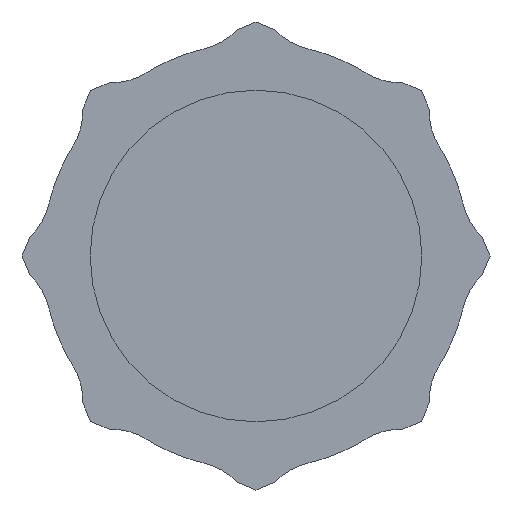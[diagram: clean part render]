
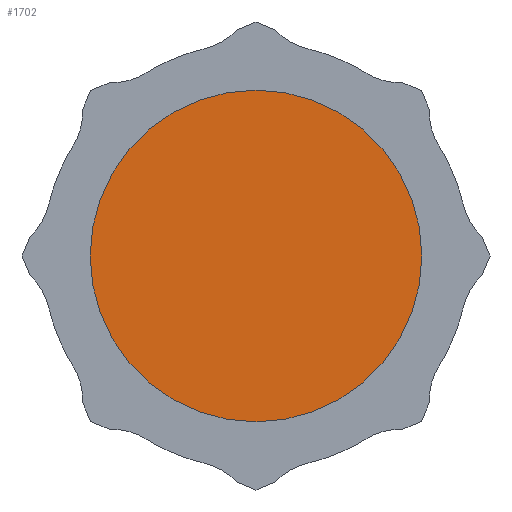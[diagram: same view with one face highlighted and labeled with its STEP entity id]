
A CAD part, front view. The second image highlights one B-rep face of the part: STEP entity #1702.
In plain terms, the highlighted planar face has unit normal (0, -1, 0).
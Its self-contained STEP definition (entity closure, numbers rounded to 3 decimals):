
#25=PLANE('',#1928);
#132=CIRCLE('',#1927,3.125);
#255=FACE_OUTER_BOUND('',#355,.T.);
#355=EDGE_LOOP('',(#1417));
#771=VERTEX_POINT('',#3386);
#1006=EDGE_CURVE('',#771,#771,#132,.T.);
#1417=ORIENTED_EDGE('',*,*,#1006,.T.);
#1702=ADVANCED_FACE('',(#255),#25,.F.);
#1927=AXIS2_PLACEMENT_3D('',#3388,#2405,#2406);
#1928=AXIS2_PLACEMENT_3D('',#3389,#2407,#2408);
#2405=DIRECTION('center_axis',(0.,-1.,0.));
#2406=DIRECTION('ref_axis',(1.,0.,0.));
#2407=DIRECTION('center_axis',(0.,1.,0.));
#2408=DIRECTION('ref_axis',(0.,0.,1.));
#3386=CARTESIAN_POINT('',(-3.125,48.26,0.));
#3388=CARTESIAN_POINT('Origin',(0.,48.26,0.));
#3389=CARTESIAN_POINT('Origin',(0.,48.26,0.));
